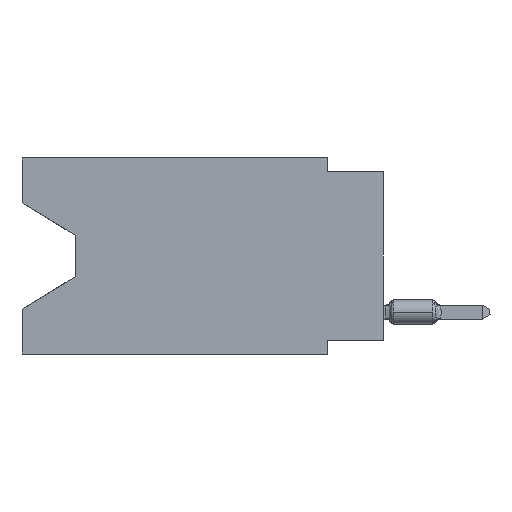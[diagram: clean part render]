
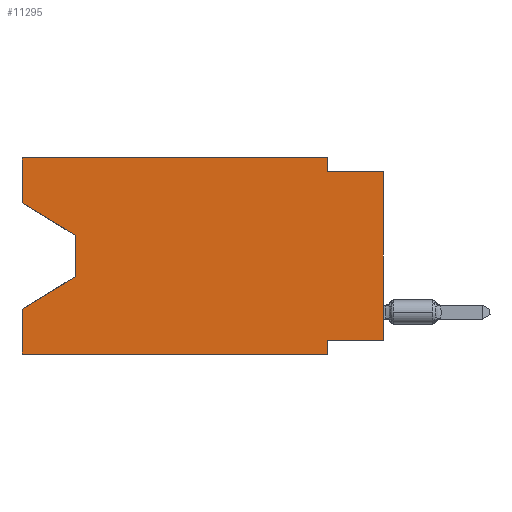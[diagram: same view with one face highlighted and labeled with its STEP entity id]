
A CAD part, left-side view. The second image highlights one B-rep face of the part: STEP entity #11295.
In plain terms, the highlighted planar face has unit normal (-1, 0, 0).
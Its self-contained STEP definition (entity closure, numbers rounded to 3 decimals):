
#755 = DIRECTION ( 'NONE',  ( 0., 0., -1. ) ) ;
#1283 = CARTESIAN_POINT ( 'NONE',  ( 0., 16.383, -2.038 ) ) ;
#1341 = ORIENTED_EDGE ( 'NONE', *, *, #29103, .T. ) ;
#1898 = VECTOR ( 'NONE', #55297, 1000. ) ;
#2430 = ORIENTED_EDGE ( 'NONE', *, *, #5637, .F. ) ;
#3385 = LINE ( 'NONE', #46793, #41619 ) ;
#4333 = DIRECTION ( 'NONE',  ( 0., -1., 0. ) ) ;
#5637 = EDGE_CURVE ( 'NONE', #35540, #67768, #7725, .T. ) ;
#5829 = CARTESIAN_POINT ( 'NONE',  ( 0., 2.54, -8.89 ) ) ;
#6525 = VECTOR ( 'NONE', #56843, 1000. ) ;
#6750 = ORIENTED_EDGE ( 'NONE', *, *, #9181, .T. ) ;
#7129 = DIRECTION ( 'NONE',  ( 0., 0., -1. ) ) ;
#7725 = LINE ( 'NONE', #8071, #6525 ) ;
#7763 = CARTESIAN_POINT ( 'NONE',  ( 0., 2.54, -0.635 ) ) ;
#8071 = CARTESIAN_POINT ( 'NONE',  ( 0., 16.383, 0. ) ) ;
#9006 = CARTESIAN_POINT ( 'NONE',  ( 0., 16.383, -8.89 ) ) ;
#9108 = CARTESIAN_POINT ( 'NONE',  ( 0., 16.383, 0. ) ) ;
#9181 = EDGE_CURVE ( 'NONE', #51309, #61611, #21902, .T. ) ;
#9342 = DIRECTION ( 'NONE',  ( 0., 1., 0. ) ) ;
#11105 = VERTEX_POINT ( 'NONE', #37746 ) ;
#11295 = ADVANCED_FACE ( 'NONE', ( #24675 ), #25034, .F. ) ;
#11714 = VECTOR ( 'NONE', #9342, 1000. ) ;
#11889 = ORIENTED_EDGE ( 'NONE', *, *, #62445, .F. ) ;
#12125 = DIRECTION ( 'NONE',  ( 0., 0.855, -0.519 ) ) ;
#13229 = EDGE_CURVE ( 'NONE', #39758, #36154, #33535, .T. ) ;
#13300 = CARTESIAN_POINT ( 'NONE',  ( 0., 16.383, 0. ) ) ;
#14653 = DIRECTION ( 'NONE',  ( 0., 0., -1. ) ) ;
#15023 = VERTEX_POINT ( 'NONE', #35467 ) ;
#15782 = LINE ( 'NONE', #9006, #63013 ) ;
#15889 = EDGE_CURVE ( 'NONE', #35540, #46703, #57190, .T. ) ;
#16178 = VECTOR ( 'NONE', #755, 1000. ) ;
#16504 = EDGE_LOOP ( 'NONE', ( #46621, #1341, #6750, #57622, #58176, #33291, #28520, #70814, #29999, #52894, #11889, #2430 ) ) ;
#16709 = VECTOR ( 'NONE', #34609, 1000. ) ;
#17125 = VECTOR ( 'NONE', #23844, 1000. ) ;
#20225 = DIRECTION ( 'NONE',  ( 0., 0., 1. ) ) ;
#21902 = LINE ( 'NONE', #56928, #66225 ) ;
#22357 = CARTESIAN_POINT ( 'NONE',  ( 0., 16.383, -8.89 ) ) ;
#22874 = CARTESIAN_POINT ( 'NONE',  ( 0., 0., -0.635 ) ) ;
#23011 = CARTESIAN_POINT ( 'NONE',  ( 0., 0., -8.255 ) ) ;
#23320 = CARTESIAN_POINT ( 'NONE',  ( 0., 2.54, 0. ) ) ;
#23844 = DIRECTION ( 'NONE',  ( 0., -0.855, -0.519 ) ) ;
#24675 = FACE_OUTER_BOUND ( 'NONE', #16504, .T. ) ;
#25034 = PLANE ( 'NONE',  #48625 ) ;
#28269 = LINE ( 'NONE', #22874, #44935 ) ;
#28520 = ORIENTED_EDGE ( 'NONE', *, *, #50759, .F. ) ;
#29103 = EDGE_CURVE ( 'NONE', #46703, #51309, #51909, .T. ) ;
#29597 = EDGE_CURVE ( 'NONE', #68533, #36154, #28269, .T. ) ;
#29999 = ORIENTED_EDGE ( 'NONE', *, *, #29597, .F. ) ;
#33291 = ORIENTED_EDGE ( 'NONE', *, *, #69167, .F. ) ;
#33535 = LINE ( 'NONE', #55429, #16709 ) ;
#34609 = DIRECTION ( 'NONE',  ( 0., 0., 1. ) ) ;
#35467 = CARTESIAN_POINT ( 'NONE',  ( 0., 2.54, 0. ) ) ;
#35514 = DIRECTION ( 'NONE',  ( 0., -1., 0. ) ) ;
#35540 = VERTEX_POINT ( 'NONE', #42447 ) ;
#36154 = VERTEX_POINT ( 'NONE', #55944 ) ;
#37393 = CARTESIAN_POINT ( 'NONE',  ( 0., 2.54, -8.255 ) ) ;
#37746 = CARTESIAN_POINT ( 'NONE',  ( 0., 2.54, -8.89 ) ) ;
#39758 = VERTEX_POINT ( 'NONE', #23011 ) ;
#40121 = EDGE_CURVE ( 'NONE', #43480, #11105, #15782, .T. ) ;
#41619 = VECTOR ( 'NONE', #20225, 1000. ) ;
#42447 = CARTESIAN_POINT ( 'NONE',  ( 0., 16.383, -2.038 ) ) ;
#42854 = EDGE_CURVE ( 'NONE', #15023, #68533, #49895, .T. ) ;
#43480 = VERTEX_POINT ( 'NONE', #22357 ) ;
#44728 = EDGE_CURVE ( 'NONE', #43480, #61611, #3385, .T. ) ;
#44775 = DIRECTION ( 'NONE',  ( 0., -1., 0. ) ) ;
#44935 = VECTOR ( 'NONE', #44775, 1000. ) ;
#46593 = DIRECTION ( 'NONE',  ( 1., 0., 0. ) ) ;
#46621 = ORIENTED_EDGE ( 'NONE', *, *, #15889, .T. ) ;
#46703 = VERTEX_POINT ( 'NONE', #70480 ) ;
#46793 = CARTESIAN_POINT ( 'NONE',  ( 0., 16.383, 0. ) ) ;
#47306 = CARTESIAN_POINT ( 'NONE',  ( 0., 16.383, 0. ) ) ;
#48089 = VECTOR ( 'NONE', #35514, 1000. ) ;
#48625 = AXIS2_PLACEMENT_3D ( 'NONE', #47306, #46593, #14653 ) ;
#49895 = LINE ( 'NONE', #23320, #16178 ) ;
#50759 = EDGE_CURVE ( 'NONE', #39758, #54786, #54148, .T. ) ;
#50791 = CARTESIAN_POINT ( 'NONE',  ( 0., 16.383, -6.852 ) ) ;
#51309 = VERTEX_POINT ( 'NONE', #65163 ) ;
#51327 = LINE ( 'NONE', #13300, #48089 ) ;
#51909 = LINE ( 'NONE', #67701, #55036 ) ;
#52894 = ORIENTED_EDGE ( 'NONE', *, *, #42854, .F. ) ;
#54148 = LINE ( 'NONE', #58101, #11714 ) ;
#54786 = VERTEX_POINT ( 'NONE', #37393 ) ;
#54947 = LINE ( 'NONE', #5829, #1898 ) ;
#55036 = VECTOR ( 'NONE', #7129, 1000. ) ;
#55297 = DIRECTION ( 'NONE',  ( 0., 0., -1. ) ) ;
#55429 = CARTESIAN_POINT ( 'NONE',  ( 0., 0., 0. ) ) ;
#55944 = CARTESIAN_POINT ( 'NONE',  ( 0., 0., -0.635 ) ) ;
#56843 = DIRECTION ( 'NONE',  ( 0., 0., 1. ) ) ;
#56928 = CARTESIAN_POINT ( 'NONE',  ( 0., 13.97, -5.385 ) ) ;
#57190 = LINE ( 'NONE', #1283, #17125 ) ;
#57622 = ORIENTED_EDGE ( 'NONE', *, *, #44728, .F. ) ;
#58101 = CARTESIAN_POINT ( 'NONE',  ( 0., 0., -8.255 ) ) ;
#58176 = ORIENTED_EDGE ( 'NONE', *, *, #40121, .T. ) ;
#61611 = VERTEX_POINT ( 'NONE', #50791 ) ;
#62445 = EDGE_CURVE ( 'NONE', #67768, #15023, #51327, .T. ) ;
#63013 = VECTOR ( 'NONE', #4333, 1000. ) ;
#65163 = CARTESIAN_POINT ( 'NONE',  ( 0., 13.97, -5.385 ) ) ;
#66225 = VECTOR ( 'NONE', #12125, 1000. ) ;
#67701 = CARTESIAN_POINT ( 'NONE',  ( 0., 13.97, -3.505 ) ) ;
#67768 = VERTEX_POINT ( 'NONE', #9108 ) ;
#68533 = VERTEX_POINT ( 'NONE', #7763 ) ;
#69167 = EDGE_CURVE ( 'NONE', #54786, #11105, #54947, .T. ) ;
#70480 = CARTESIAN_POINT ( 'NONE',  ( 0., 13.97, -3.505 ) ) ;
#70814 = ORIENTED_EDGE ( 'NONE', *, *, #13229, .T. ) ;
